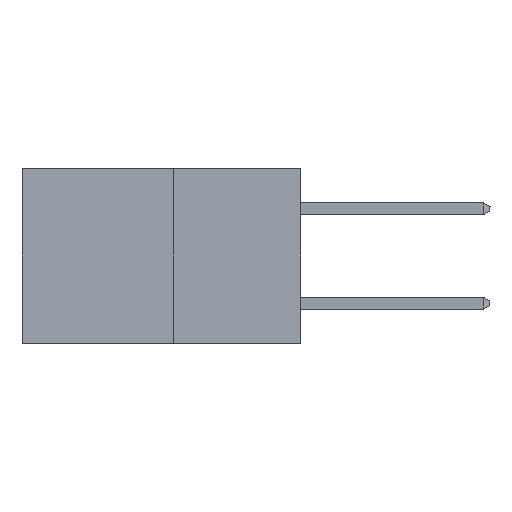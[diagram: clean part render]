
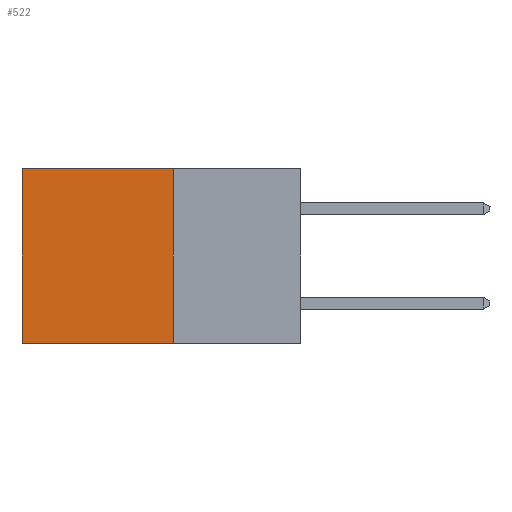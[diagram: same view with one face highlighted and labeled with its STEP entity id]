
A CAD part, left-side view. The second image highlights one B-rep face of the part: STEP entity #522.
In plain terms, the highlighted planar face has unit normal (-1, 0, 0).
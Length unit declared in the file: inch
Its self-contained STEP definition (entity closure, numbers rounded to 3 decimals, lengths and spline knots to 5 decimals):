
#522 = ADVANCED_FACE ( 'NONE', ( #10403 ), #1024, .F. ) ;
#838 = LINE ( 'NONE', #4781, #11041 ) ;
#906 = DIRECTION ( 'NONE',  ( 1., 0., 0. ) ) ;
#1024 = PLANE ( 'NONE',  #9557 ) ;
#1237 = EDGE_CURVE ( 'NONE', #2001, #2865, #838, .T. ) ;
#2001 = VERTEX_POINT ( 'NONE', #10482 ) ;
#2156 = CARTESIAN_POINT ( 'NONE',  ( 0.277, 0.59, -0.37 ) ) ;
#2834 = VECTOR ( 'NONE', #9500, 39.37008 ) ;
#2865 = VERTEX_POINT ( 'NONE', #6186 ) ;
#3775 = VECTOR ( 'NONE', #3922, 39.37008 ) ;
#3922 = DIRECTION ( 'NONE',  ( 0., 0., -1. ) ) ;
#4169 = EDGE_CURVE ( 'NONE', #11432, #5514, #8068, .T. ) ;
#4280 = ORIENTED_EDGE ( 'NONE', *, *, #1237, .T. ) ;
#4710 = LINE ( 'NONE', #9756, #3775 ) ;
#4781 = CARTESIAN_POINT ( 'NONE',  ( 0.277, 0.27, 0. ) ) ;
#5514 = VERTEX_POINT ( 'NONE', #2156 ) ;
#6186 = CARTESIAN_POINT ( 'NONE',  ( 0.277, 0.59, 0. ) ) ;
#6508 = EDGE_CURVE ( 'NONE', #2001, #11432, #9159, .T. ) ;
#7227 = CARTESIAN_POINT ( 'NONE',  ( 0.277, 0.27, -0.37 ) ) ;
#7794 = DIRECTION ( 'NONE',  ( 0., 0., -1. ) ) ;
#7899 = EDGE_CURVE ( 'NONE', #2865, #5514, #4710, .T. ) ;
#8068 = LINE ( 'NONE', #11656, #2834 ) ;
#8126 = EDGE_LOOP ( 'NONE', ( #8413, #10982, #12297, #4280 ) ) ;
#8413 = ORIENTED_EDGE ( 'NONE', *, *, #7899, .T. ) ;
#8501 = CARTESIAN_POINT ( 'NONE',  ( 0.277, 0.27, -0.37 ) ) ;
#9159 = LINE ( 'NONE', #10001, #11428 ) ;
#9500 = DIRECTION ( 'NONE',  ( 0., 1., 0. ) ) ;
#9557 = AXIS2_PLACEMENT_3D ( 'NONE', #7227, #906, #7794 ) ;
#9756 = CARTESIAN_POINT ( 'NONE',  ( 0.277, 0.59, -0.37 ) ) ;
#10001 = CARTESIAN_POINT ( 'NONE',  ( 0.277, 0.27, -0.37 ) ) ;
#10062 = DIRECTION ( 'NONE',  ( 0., 0., -1. ) ) ;
#10403 = FACE_OUTER_BOUND ( 'NONE', #8126, .T. ) ;
#10482 = CARTESIAN_POINT ( 'NONE',  ( 0.277, 0.27, 0. ) ) ;
#10982 = ORIENTED_EDGE ( 'NONE', *, *, #4169, .F. ) ;
#11041 = VECTOR ( 'NONE', #12346, 39.37008 ) ;
#11428 = VECTOR ( 'NONE', #10062, 39.37008 ) ;
#11432 = VERTEX_POINT ( 'NONE', #8501 ) ;
#11656 = CARTESIAN_POINT ( 'NONE',  ( 0.277, 0.27, -0.37 ) ) ;
#12297 = ORIENTED_EDGE ( 'NONE', *, *, #6508, .F. ) ;
#12346 = DIRECTION ( 'NONE',  ( 0., 1., 0. ) ) ;
